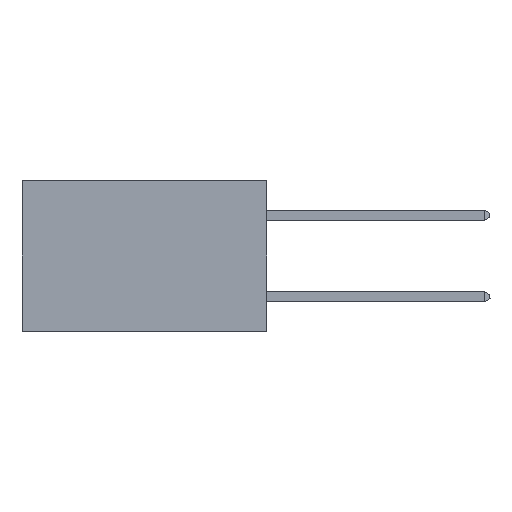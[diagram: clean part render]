
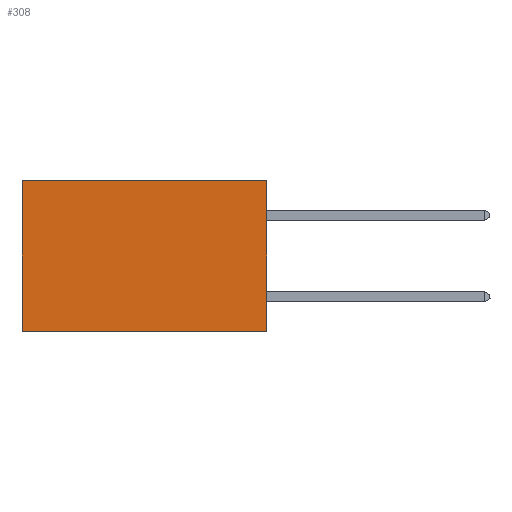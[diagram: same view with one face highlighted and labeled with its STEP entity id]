
A CAD part, left-side view. The second image highlights one B-rep face of the part: STEP entity #308.
In plain terms, the highlighted planar face has unit normal (-1, 0, 0).
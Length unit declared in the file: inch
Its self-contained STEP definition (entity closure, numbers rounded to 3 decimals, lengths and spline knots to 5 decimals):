
#308 = ADVANCED_FACE ( 'NONE', ( #10177 ), #26471, .F. ) ;
#484 = CARTESIAN_POINT ( 'NONE',  ( 0.2875, 0.6, 0. ) ) ;
#1465 = ORIENTED_EDGE ( 'NONE', *, *, #31390, .T. ) ;
#3793 = ORIENTED_EDGE ( 'NONE', *, *, #8768, .T. ) ;
#4181 = DIRECTION ( 'NONE',  ( 0., 0., -1. ) ) ;
#5887 = ORIENTED_EDGE ( 'NONE', *, *, #21324, .F. ) ;
#6164 = DIRECTION ( 'NONE',  ( 0., 0., -1. ) ) ;
#6739 = CARTESIAN_POINT ( 'NONE',  ( 0.2875, 0., 0. ) ) ;
#6880 = VECTOR ( 'NONE', #6164, 39.37008 ) ;
#7418 = CARTESIAN_POINT ( 'NONE',  ( 0.2875, 0., 0. ) ) ;
#7432 = AXIS2_PLACEMENT_3D ( 'NONE', #29304, #35574, #4181 ) ;
#8768 = EDGE_CURVE ( 'NONE', #12910, #21134, #13645, .T. ) ;
#10177 = FACE_OUTER_BOUND ( 'NONE', #19248, .T. ) ;
#11061 = VECTOR ( 'NONE', #15847, 39.37008 ) ;
#11317 = CARTESIAN_POINT ( 'NONE',  ( 0.2875, 0., 0. ) ) ;
#12125 = LINE ( 'NONE', #11317, #26314 ) ;
#12148 = VERTEX_POINT ( 'NONE', #23959 ) ;
#12557 = CARTESIAN_POINT ( 'NONE',  ( 0.2875, 0., -0.37 ) ) ;
#12687 = LINE ( 'NONE', #484, #6880 ) ;
#12910 = VERTEX_POINT ( 'NONE', #7418 ) ;
#13645 = LINE ( 'NONE', #6739, #26009 ) ;
#15485 = ORIENTED_EDGE ( 'NONE', *, *, #30732, .F. ) ;
#15847 = DIRECTION ( 'NONE',  ( 0., 1., 0. ) ) ;
#19248 = EDGE_LOOP ( 'NONE', ( #1465, #5887, #15485, #3793 ) ) ;
#21134 = VERTEX_POINT ( 'NONE', #22336 ) ;
#21324 = EDGE_CURVE ( 'NONE', #24188, #12148, #31860, .T. ) ;
#22336 = CARTESIAN_POINT ( 'NONE',  ( 0.2875, 0.6, 0. ) ) ;
#23959 = CARTESIAN_POINT ( 'NONE',  ( 0.2875, 0.6, -0.37 ) ) ;
#24188 = VERTEX_POINT ( 'NONE', #12557 ) ;
#26009 = VECTOR ( 'NONE', #29525, 39.37008 ) ;
#26314 = VECTOR ( 'NONE', #28765, 39.37008 ) ;
#26471 = PLANE ( 'NONE',  #7432 ) ;
#28765 = DIRECTION ( 'NONE',  ( 0., 0., -1. ) ) ;
#29304 = CARTESIAN_POINT ( 'NONE',  ( 0.2875, 0., 0. ) ) ;
#29525 = DIRECTION ( 'NONE',  ( 0., 1., 0. ) ) ;
#30732 = EDGE_CURVE ( 'NONE', #12910, #24188, #12125, .T. ) ;
#31390 = EDGE_CURVE ( 'NONE', #21134, #12148, #12687, .T. ) ;
#31860 = LINE ( 'NONE', #32952, #11061 ) ;
#32952 = CARTESIAN_POINT ( 'NONE',  ( 0.2875, 0., -0.37 ) ) ;
#35574 = DIRECTION ( 'NONE',  ( 1., 0., 0. ) ) ;
